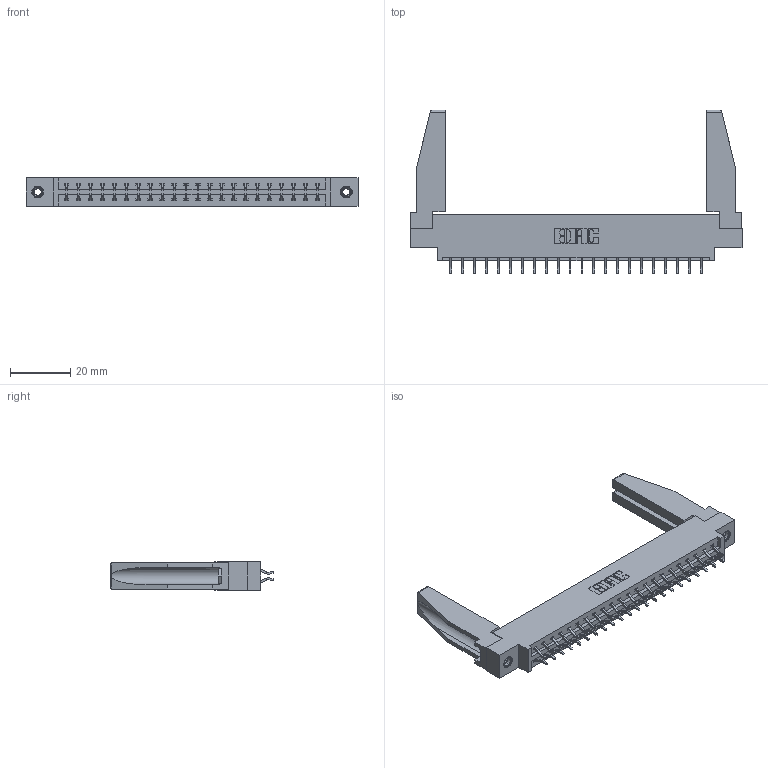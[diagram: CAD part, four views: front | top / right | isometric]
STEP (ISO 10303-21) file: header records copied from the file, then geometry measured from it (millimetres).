
FILE_DESCRIPTION (( 'STEP AP203' ), '1' );
FILE_NAME ('387-044-556-878.STEP', '2019-10-18T06:24:58', ( '' ), ( '' ), 'SwSTEP 2.0', 'SolidWorks 2016', '' );
FILE_SCHEMA (( 'CONFIG_CONTROL_DESIGN' ));
Length unit declared in the file: inch
Products named in the file (5): 345-292-001_556 Tail; 345-250-001_345-250-001-102; 337 Part_0.170 Offset - 0.156 Dia-TI; 307-220-078; 387-044-556-878
Assembly tree (49 placements, depth 2):
  387-044-556-878
    337 Part_0.170 Offset - 0.156 Dia-TI
    345-292-001_556 Tail  x44
    345-250-001_345-250-001-102  x2
    307-220-078  x2
Bounding box: 110.19 x 54.37 x 9.4 mm (x, y, z)
Volume: 15220.1 mm3; surface area: 16389.4 mm2
Topology: 49 solids, 49 shells, 2888 faces, 8529 edges, 5618 vertices
Faces by surface type: plane 2006, cylinder 866, cone 12, torus 4
Entity records: 22436 total; most frequent: CARTESIAN_POINT 3812, ORIENTED_EDGE 3692, DIRECTION 3274, EDGE_CURVE 1846, VECTOR 1672, LINE 1672, VERTEX_POINT 1224, AXIS2_PLACEMENT_3D 801
